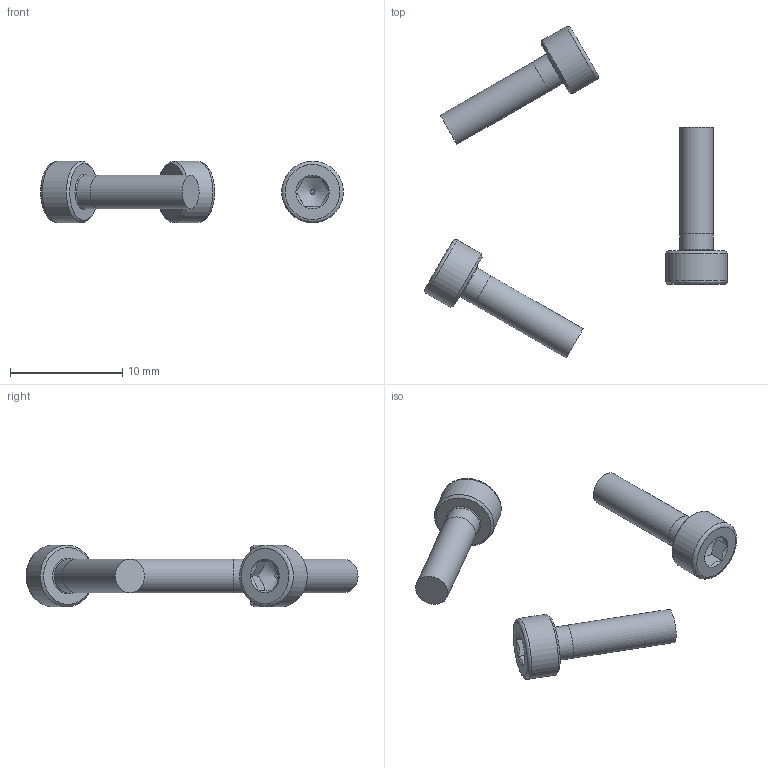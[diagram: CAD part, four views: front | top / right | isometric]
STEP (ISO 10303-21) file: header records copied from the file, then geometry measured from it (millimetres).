
FILE_DESCRIPTION(('FreeCAD Model'),'2;1');
FILE_NAME('Open CASCADE Shape Model','2022-10-05T16:42:15',('Author'),( ''),'Open CASCADE STEP processor 7.6','FreeCAD','Unknown');
FILE_SCHEMA(('AUTOMOTIVE_DESIGN { 1 0 10303 214 1 1 1 1 }'));
Length unit declared in the file: millimetre
Products named in the file (1): m3 screws
Bounding box: 27.01 x 29.62 x 5.5 mm (x, y, z)
Volume: 416.1 mm3; surface area: 632.5 mm2
Topology: 3 solids, 3 shells, 54 faces, 114 edges, 69 vertices
Faces by surface type: plane 27, cone 9, cylinder 9, revolution 6, sphere 3
Full cylindrical faces by diameter (mm): 3 x6, 5.5 x3
Entity records: 3263 total; most frequent: CARTESIAN_POINT 931, DIRECTION 452, ORIENTED_EDGE 222, PCURVE 222, DEFINITIONAL_REPRESENTATION 222, LINE 171, VECTOR 171, AXIS2_PLACEMENT_3D 130
